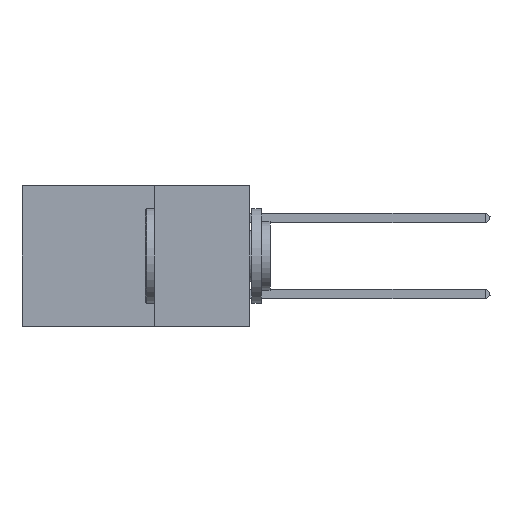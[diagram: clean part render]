
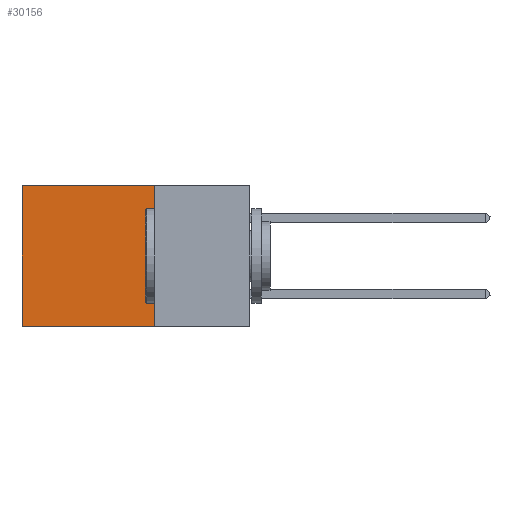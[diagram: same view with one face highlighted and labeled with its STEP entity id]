
A CAD part, left-side view. The second image highlights one B-rep face of the part: STEP entity #30156.
In plain terms, the highlighted planar face has unit normal (-1, 0, 0).
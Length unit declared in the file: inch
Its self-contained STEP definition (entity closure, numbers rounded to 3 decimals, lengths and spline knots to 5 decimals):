
#381 = VERTEX_POINT ( 'NONE', #956 ) ;
#723 = VECTOR ( 'NONE', #6008, 39.37008 ) ;
#956 = CARTESIAN_POINT ( 'NONE',  ( 0.2875, 0.6, -0.37 ) ) ;
#3506 = AXIS2_PLACEMENT_3D ( 'NONE', #26623, #16378, #13872 ) ;
#6008 = DIRECTION ( 'NONE',  ( 0., 1., 0. ) ) ;
#6067 = ORIENTED_EDGE ( 'NONE', *, *, #13220, .F. ) ;
#8008 = CARTESIAN_POINT ( 'NONE',  ( 0.2875, 0.6, 0. ) ) ;
#8379 = LINE ( 'NONE', #8646, #18934 ) ;
#8536 = FACE_OUTER_BOUND ( 'NONE', #16682, .T. ) ;
#8646 = CARTESIAN_POINT ( 'NONE',  ( 0.2875, 0.25, -0.37 ) ) ;
#10056 = LINE ( 'NONE', #8008, #18154 ) ;
#11205 = EDGE_CURVE ( 'NONE', #21037, #27377, #17027, .T. ) ;
#12766 = ORIENTED_EDGE ( 'NONE', *, *, #16923, .T. ) ;
#13220 = EDGE_CURVE ( 'NONE', #27377, #381, #8379, .T. ) ;
#13654 = PLANE ( 'NONE',  #3506 ) ;
#13872 = DIRECTION ( 'NONE',  ( 0., 0., -1. ) ) ;
#16378 = DIRECTION ( 'NONE',  ( 1., 0., 0. ) ) ;
#16682 = EDGE_LOOP ( 'NONE', ( #21157, #6067, #27059, #12766 ) ) ;
#16923 = EDGE_CURVE ( 'NONE', #21037, #23607, #22734, .T. ) ;
#17027 = LINE ( 'NONE', #20433, #30459 ) ;
#17865 = CARTESIAN_POINT ( 'NONE',  ( 0.2875, 0.6, 0. ) ) ;
#18154 = VECTOR ( 'NONE', #18437, 39.37008 ) ;
#18437 = DIRECTION ( 'NONE',  ( 0., 0., -1. ) ) ;
#18934 = VECTOR ( 'NONE', #29738, 39.37008 ) ;
#20399 = CARTESIAN_POINT ( 'NONE',  ( 0.2875, 0.25, -0.37 ) ) ;
#20433 = CARTESIAN_POINT ( 'NONE',  ( 0.2875, 0.25, 0. ) ) ;
#21037 = VERTEX_POINT ( 'NONE', #27349 ) ;
#21157 = ORIENTED_EDGE ( 'NONE', *, *, #23741, .T. ) ;
#21593 = CARTESIAN_POINT ( 'NONE',  ( 0.2875, 0.25, 0. ) ) ;
#22734 = LINE ( 'NONE', #21593, #723 ) ;
#23607 = VERTEX_POINT ( 'NONE', #17865 ) ;
#23741 = EDGE_CURVE ( 'NONE', #23607, #381, #10056, .T. ) ;
#25869 = DIRECTION ( 'NONE',  ( 0., 0., -1. ) ) ;
#26623 = CARTESIAN_POINT ( 'NONE',  ( 0.2875, 0.25, 0. ) ) ;
#27059 = ORIENTED_EDGE ( 'NONE', *, *, #11205, .F. ) ;
#27349 = CARTESIAN_POINT ( 'NONE',  ( 0.2875, 0.25, 0. ) ) ;
#27377 = VERTEX_POINT ( 'NONE', #20399 ) ;
#29738 = DIRECTION ( 'NONE',  ( 0., 1., 0. ) ) ;
#30156 = ADVANCED_FACE ( 'NONE', ( #8536 ), #13654, .F. ) ;
#30459 = VECTOR ( 'NONE', #25869, 39.37008 ) ;
